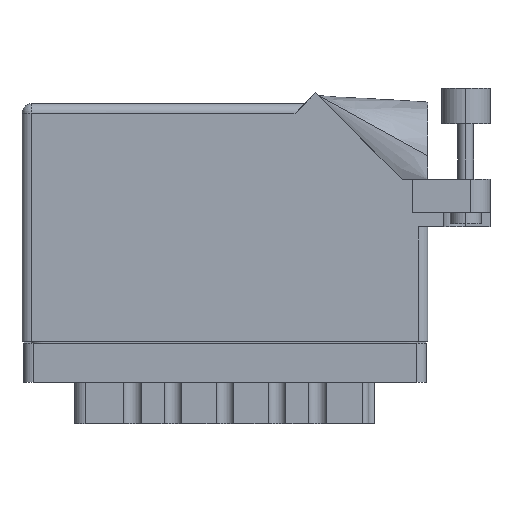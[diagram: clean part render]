
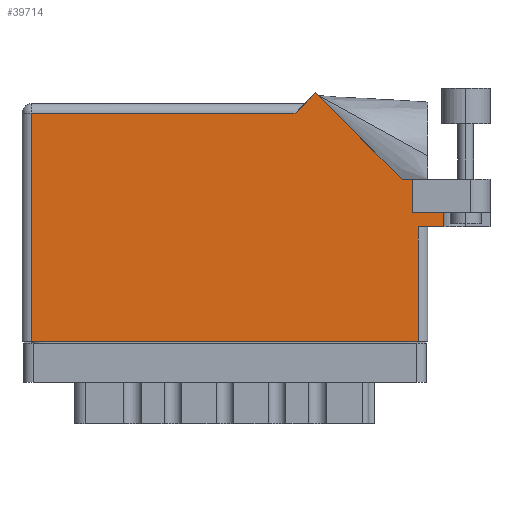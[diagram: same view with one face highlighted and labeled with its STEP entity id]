
A CAD part, front view. The second image highlights one B-rep face of the part: STEP entity #39714.
In plain terms, the highlighted face is planar.
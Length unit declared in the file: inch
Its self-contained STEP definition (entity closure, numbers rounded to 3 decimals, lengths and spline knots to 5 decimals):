
#572 = LINE ( 'NONE', #27724, #49497 ) ;
#689 = CARTESIAN_POINT ( 'NONE',  ( 1.88971, 1.60071, 0. ) ) ;
#1131 = CARTESIAN_POINT ( 'NONE',  ( 0.062, 0., 0. ) ) ;
#1445 = EDGE_LOOP ( 'NONE', ( #6888, #23063, #22624, #7954, #14126, #36642, #33587, #38260, #4167, #48620, #14159 ) ) ;
#1515 = CARTESIAN_POINT ( 'NONE',  ( 0., 1.468, 0. ) ) ;
#2571 = VERTEX_POINT ( 'NONE', #39673 ) ;
#2754 = VERTEX_POINT ( 'NONE', #20879 ) ;
#2907 = VECTOR ( 'NONE', #18084, 39.37008 ) ;
#4167 = ORIENTED_EDGE ( 'NONE', *, *, #28589, .T. ) ;
#4250 = DIRECTION ( 'NONE',  ( -1., 0., 0. ) ) ;
#4890 = CARTESIAN_POINT ( 'NONE',  ( 2.512, 1.044, 0. ) ) ;
#4980 = LINE ( 'NONE', #26345, #47293 ) ;
#6888 = ORIENTED_EDGE ( 'NONE', *, *, #50050, .T. ) ;
#7570 = DIRECTION ( 'NONE',  ( -0.707, 0.707, 0. ) ) ;
#7954 = ORIENTED_EDGE ( 'NONE', *, *, #49862, .F. ) ;
#9099 = VECTOR ( 'NONE', #28819, 39.37008 ) ;
#9653 = LINE ( 'NONE', #20178, #12677 ) ;
#9772 = VERTEX_POINT ( 'NONE', #17370 ) ;
#9849 = VERTEX_POINT ( 'NONE', #1131 ) ;
#11754 = CARTESIAN_POINT ( 'NONE',  ( 2.44642, 1.044, 0. ) ) ;
#12200 = CARTESIAN_POINT ( 'NONE',  ( 2.55, 0.737, 0. ) ) ;
#12663 = PLANE ( 'NONE',  #16674 ) ;
#12677 = VECTOR ( 'NONE', #40964, 39.37008 ) ;
#13941 = EDGE_CURVE ( 'NONE', #9772, #9849, #4980, .T. ) ;
#14126 = ORIENTED_EDGE ( 'NONE', *, *, #29736, .F. ) ;
#14159 = ORIENTED_EDGE ( 'NONE', *, *, #13941, .T. ) ;
#14473 = DIRECTION ( 'NONE',  ( 0., 1., 0. ) ) ;
#14638 = VERTEX_POINT ( 'NONE', #12200 ) ;
#14750 = DIRECTION ( 'NONE',  ( -0.707, -0.707, 0. ) ) ;
#15023 = LINE ( 'NONE', #38917, #42217 ) ;
#15396 = VERTEX_POINT ( 'NONE', #33100 ) ;
#15969 = LINE ( 'NONE', #24701, #48639 ) ;
#16450 = VECTOR ( 'NONE', #31949, 39.37008 ) ;
#16674 = AXIS2_PLACEMENT_3D ( 'NONE', #27383, #19884, #4250 ) ;
#17167 = LINE ( 'NONE', #49216, #48651 ) ;
#17370 = CARTESIAN_POINT ( 'NONE',  ( 0.062, 1.468, 0. ) ) ;
#18084 = DIRECTION ( 'NONE',  ( 1., 0., 0. ) ) ;
#18209 = EDGE_CURVE ( 'NONE', #18515, #2754, #572, .T. ) ;
#18515 = VERTEX_POINT ( 'NONE', #4890 ) ;
#18862 = LINE ( 'NONE', #32113, #16450 ) ;
#19336 = VERTEX_POINT ( 'NONE', #689 ) ;
#19884 = DIRECTION ( 'NONE',  ( 0., 0., -1. ) ) ;
#20178 = CARTESIAN_POINT ( 'NONE',  ( 2.55, 0.737, 0. ) ) ;
#20354 = FACE_OUTER_BOUND ( 'NONE', #1445, .T. ) ;
#20879 = CARTESIAN_POINT ( 'NONE',  ( 2.44642, 1.044, 0. ) ) ;
#22624 = ORIENTED_EDGE ( 'NONE', *, *, #35200, .T. ) ;
#23063 = ORIENTED_EDGE ( 'NONE', *, *, #48206, .T. ) ;
#23442 = LINE ( 'NONE', #25210, #2907 ) ;
#23665 = DIRECTION ( 'NONE',  ( -1., 0., 0. ) ) ;
#23749 = CARTESIAN_POINT ( 'NONE',  ( 2.55, 0., 0. ) ) ;
#24512 = VECTOR ( 'NONE', #14473, 39.37008 ) ;
#24701 = CARTESIAN_POINT ( 'NONE',  ( 2.612, 0.737, 0. ) ) ;
#24854 = DIRECTION ( 'NONE',  ( 1., 0., 0. ) ) ;
#25210 = CARTESIAN_POINT ( 'NONE',  ( 0., 0., 0. ) ) ;
#25481 = EDGE_CURVE ( 'NONE', #2754, #19336, #32996, .T. ) ;
#26037 = LINE ( 'NONE', #1515, #9099 ) ;
#26345 = CARTESIAN_POINT ( 'NONE',  ( 0.062, 0., 0. ) ) ;
#27383 = CARTESIAN_POINT ( 'NONE',  ( 0., 1.53, 0. ) ) ;
#27724 = CARTESIAN_POINT ( 'NONE',  ( 3.012, 1.044, 0. ) ) ;
#28589 = EDGE_CURVE ( 'NONE', #19336, #2571, #17167, .T. ) ;
#28819 = DIRECTION ( 'NONE',  ( -1., 0., 0. ) ) ;
#29412 = VERTEX_POINT ( 'NONE', #44151 ) ;
#29736 = EDGE_CURVE ( 'NONE', #35438, #15396, #18862, .T. ) ;
#30160 = CARTESIAN_POINT ( 'NONE',  ( 2.512, 0.831, 0. ) ) ;
#31551 = EDGE_CURVE ( 'NONE', #2571, #9772, #26037, .T. ) ;
#31949 = DIRECTION ( 'NONE',  ( 1., 0., 0. ) ) ;
#32113 = CARTESIAN_POINT ( 'NONE',  ( 2.512, 0.831, 0. ) ) ;
#32996 = LINE ( 'NONE', #11754, #43316 ) ;
#33100 = CARTESIAN_POINT ( 'NONE',  ( 2.7135, 0.831, 0. ) ) ;
#33587 = ORIENTED_EDGE ( 'NONE', *, *, #18209, .T. ) ;
#34153 = LINE ( 'NONE', #30160, #24512 ) ;
#35036 = EDGE_CURVE ( 'NONE', #35438, #18515, #34153, .T. ) ;
#35200 = EDGE_CURVE ( 'NONE', #14638, #29412, #15969, .T. ) ;
#35438 = VERTEX_POINT ( 'NONE', #49696 ) ;
#36642 = ORIENTED_EDGE ( 'NONE', *, *, #35036, .T. ) ;
#38260 = ORIENTED_EDGE ( 'NONE', *, *, #25481, .T. ) ;
#38917 = CARTESIAN_POINT ( 'NONE',  ( 2.7135, 1.16177, 0. ) ) ;
#39086 = DIRECTION ( 'NONE',  ( 0., -1., 0. ) ) ;
#39673 = CARTESIAN_POINT ( 'NONE',  ( 1.757, 1.468, 0. ) ) ;
#39714 = ADVANCED_FACE ( 'NONE', ( #20354 ), #12663, .F. ) ;
#40964 = DIRECTION ( 'NONE',  ( 0., 1., 0. ) ) ;
#41183 = DIRECTION ( 'NONE',  ( 0., -1., 0. ) ) ;
#41485 = VERTEX_POINT ( 'NONE', #23749 ) ;
#42217 = VECTOR ( 'NONE', #39086, 39.37008 ) ;
#43316 = VECTOR ( 'NONE', #7570, 39.37008 ) ;
#44151 = CARTESIAN_POINT ( 'NONE',  ( 2.7135, 0.737, 0. ) ) ;
#47293 = VECTOR ( 'NONE', #41183, 39.37008 ) ;
#48206 = EDGE_CURVE ( 'NONE', #41485, #14638, #9653, .T. ) ;
#48620 = ORIENTED_EDGE ( 'NONE', *, *, #31551, .T. ) ;
#48639 = VECTOR ( 'NONE', #24854, 39.37008 ) ;
#48651 = VECTOR ( 'NONE', #14750, 39.37008 ) ;
#49216 = CARTESIAN_POINT ( 'NONE',  ( 1.819, 1.53, 0. ) ) ;
#49497 = VECTOR ( 'NONE', #23665, 39.37008 ) ;
#49696 = CARTESIAN_POINT ( 'NONE',  ( 2.512, 0.831, 0. ) ) ;
#49862 = EDGE_CURVE ( 'NONE', #15396, #29412, #15023, .T. ) ;
#50050 = EDGE_CURVE ( 'NONE', #9849, #41485, #23442, .T. ) ;
